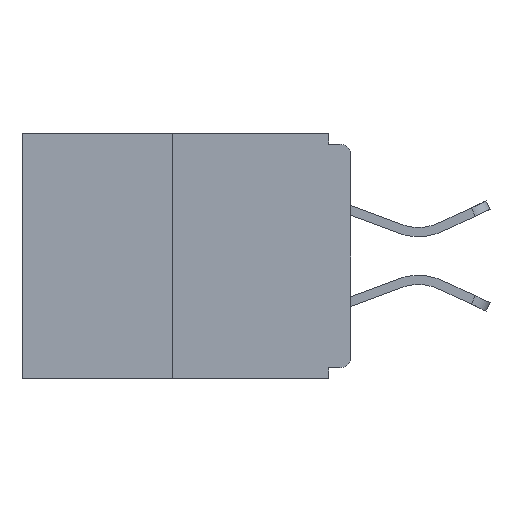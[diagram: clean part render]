
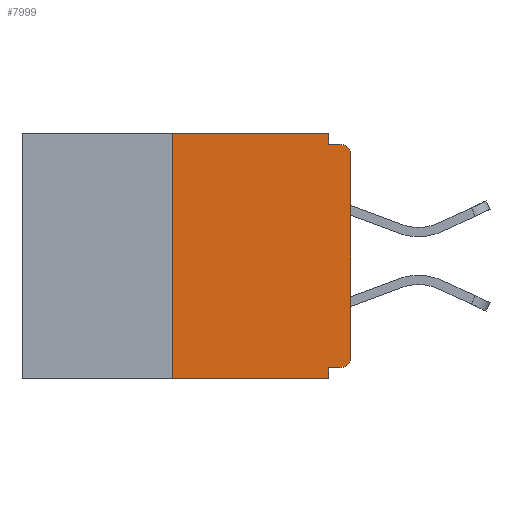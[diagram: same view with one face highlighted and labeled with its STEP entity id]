
A CAD part, left-side view. The second image highlights one B-rep face of the part: STEP entity #7999.
In plain terms, the highlighted planar face has unit normal (-1, 0, 0).
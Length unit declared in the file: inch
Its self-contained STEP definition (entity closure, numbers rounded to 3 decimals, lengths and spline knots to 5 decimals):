
#381 = CARTESIAN_POINT ( 'NONE',  ( 0., 0., 0. ) ) ;
#483 = EDGE_CURVE ( 'NONE', #3316, #15948, #10202, .T. ) ;
#600 = DIRECTION ( 'NONE',  ( -1., 0., 0. ) ) ;
#692 = LINE ( 'NONE', #10729, #14677 ) ;
#743 = CARTESIAN_POINT ( 'NONE',  ( 0., 0., -0.03 ) ) ;
#961 = ORIENTED_EDGE ( 'NONE', *, *, #10037, .F. ) ;
#969 = AXIS2_PLACEMENT_3D ( 'NONE', #8004, #9187, #3056 ) ;
#1356 = CIRCLE ( 'NONE', #11951, 0.015 ) ;
#1617 = VECTOR ( 'NONE', #6879, 39.37008 ) ;
#1692 = CARTESIAN_POINT ( 'NONE',  ( 0., 0.25, 0. ) ) ;
#2631 = DIRECTION ( 'NONE',  ( 0., -1., 0. ) ) ;
#2662 = ORIENTED_EDGE ( 'NONE', *, *, #15430, .T. ) ;
#3056 = DIRECTION ( 'NONE',  ( 0., 0., -1. ) ) ;
#3062 = EDGE_CURVE ( 'NONE', #14717, #14843, #15489, .T. ) ;
#3171 = LINE ( 'NONE', #15654, #1617 ) ;
#3316 = VERTEX_POINT ( 'NONE', #9797 ) ;
#3442 = EDGE_CURVE ( 'NONE', #5687, #5184, #4719, .T. ) ;
#4093 = VERTEX_POINT ( 'NONE', #1692 ) ;
#4639 = DIRECTION ( 'NONE',  ( 0., 0., -1. ) ) ;
#4719 = LINE ( 'NONE', #381, #10356 ) ;
#4804 = ORIENTED_EDGE ( 'NONE', *, *, #483, .T. ) ;
#5184 = VERTEX_POINT ( 'NONE', #743 ) ;
#5310 = CARTESIAN_POINT ( 'NONE',  ( 0., 0.031, -0.015 ) ) ;
#5315 = DIRECTION ( 'NONE',  ( 0., -1., 0. ) ) ;
#5323 = ORIENTED_EDGE ( 'NONE', *, *, #12602, .F. ) ;
#5418 = CARTESIAN_POINT ( 'NONE',  ( 0., 0.46, -0.343 ) ) ;
#5457 = VECTOR ( 'NONE', #2631, 39.37008 ) ;
#5539 = EDGE_CURVE ( 'NONE', #5184, #14843, #1356, .T. ) ;
#5683 = CIRCLE ( 'NONE', #969, 0.015 ) ;
#5687 = VERTEX_POINT ( 'NONE', #11135 ) ;
#6477 = CARTESIAN_POINT ( 'NONE',  ( 0., 0.031, -0.343 ) ) ;
#6554 = CARTESIAN_POINT ( 'NONE',  ( 0., 0., -0.328 ) ) ;
#6836 = ORIENTED_EDGE ( 'NONE', *, *, #5539, .T. ) ;
#6879 = DIRECTION ( 'NONE',  ( 0., 0., -1. ) ) ;
#7181 = CARTESIAN_POINT ( 'NONE',  ( 0., 0.015, -0.328 ) ) ;
#7655 = VECTOR ( 'NONE', #10045, 39.37008 ) ;
#7786 = CARTESIAN_POINT ( 'NONE',  ( 0., 0.46, 0. ) ) ;
#7956 = DIRECTION ( 'NONE',  ( 0., 0., -1. ) ) ;
#7999 = ADVANCED_FACE ( 'NONE', ( #14694 ), #13036, .F. ) ;
#8004 = CARTESIAN_POINT ( 'NONE',  ( 0., 0.015, -0.313 ) ) ;
#8194 = VECTOR ( 'NONE', #14007, 39.37008 ) ;
#8277 = CARTESIAN_POINT ( 'NONE',  ( 0., 0.031, 0. ) ) ;
#9087 = CARTESIAN_POINT ( 'NONE',  ( 0., 0., -0.015 ) ) ;
#9134 = EDGE_LOOP ( 'NONE', ( #5323, #9740, #4804, #13266, #10507, #2662, #14422, #6836, #13509, #961 ) ) ;
#9187 = DIRECTION ( 'NONE',  ( -1., 0., 0. ) ) ;
#9358 = VERTEX_POINT ( 'NONE', #13633 ) ;
#9740 = ORIENTED_EDGE ( 'NONE', *, *, #10738, .F. ) ;
#9797 = CARTESIAN_POINT ( 'NONE',  ( 0., 0.25, -0.343 ) ) ;
#10026 = DIRECTION ( 'NONE',  ( 0., 0., 1. ) ) ;
#10037 = EDGE_CURVE ( 'NONE', #13967, #14717, #692, .T. ) ;
#10045 = DIRECTION ( 'NONE',  ( 0., -1., 0. ) ) ;
#10202 = LINE ( 'NONE', #5418, #13933 ) ;
#10356 = VECTOR ( 'NONE', #12655, 39.37008 ) ;
#10507 = ORIENTED_EDGE ( 'NONE', *, *, #14682, .F. ) ;
#10713 = LINE ( 'NONE', #6554, #8194 ) ;
#10729 = CARTESIAN_POINT ( 'NONE',  ( 0., 0.031, 0. ) ) ;
#10738 = EDGE_CURVE ( 'NONE', #3316, #4093, #11344, .T. ) ;
#11135 = CARTESIAN_POINT ( 'NONE',  ( 0., 0., -0.313 ) ) ;
#11216 = CARTESIAN_POINT ( 'NONE',  ( 0., 0.25, 0. ) ) ;
#11344 = LINE ( 'NONE', #11216, #15078 ) ;
#11631 = DIRECTION ( 'NONE',  ( 1., 0., 0. ) ) ;
#11951 = AXIS2_PLACEMENT_3D ( 'NONE', #13206, #600, #14296 ) ;
#12235 = CARTESIAN_POINT ( 'NONE',  ( 0., 0.015, -0.015 ) ) ;
#12602 = EDGE_CURVE ( 'NONE', #4093, #13967, #13630, .T. ) ;
#12655 = DIRECTION ( 'NONE',  ( 0., 0., 1. ) ) ;
#13036 = PLANE ( 'NONE',  #15024 ) ;
#13073 = VERTEX_POINT ( 'NONE', #7181 ) ;
#13206 = CARTESIAN_POINT ( 'NONE',  ( 0., 0.015, -0.03 ) ) ;
#13266 = ORIENTED_EDGE ( 'NONE', *, *, #15551, .F. ) ;
#13509 = ORIENTED_EDGE ( 'NONE', *, *, #3062, .F. ) ;
#13630 = LINE ( 'NONE', #15101, #5457 ) ;
#13633 = CARTESIAN_POINT ( 'NONE',  ( 0., 0.031, -0.328 ) ) ;
#13933 = VECTOR ( 'NONE', #5315, 39.37008 ) ;
#13967 = VERTEX_POINT ( 'NONE', #8277 ) ;
#14007 = DIRECTION ( 'NONE',  ( 0., 1., 0. ) ) ;
#14296 = DIRECTION ( 'NONE',  ( 0., 0., -1. ) ) ;
#14422 = ORIENTED_EDGE ( 'NONE', *, *, #3442, .T. ) ;
#14677 = VECTOR ( 'NONE', #4639, 39.37008 ) ;
#14682 = EDGE_CURVE ( 'NONE', #13073, #9358, #10713, .T. ) ;
#14694 = FACE_OUTER_BOUND ( 'NONE', #9134, .T. ) ;
#14717 = VERTEX_POINT ( 'NONE', #5310 ) ;
#14843 = VERTEX_POINT ( 'NONE', #12235 ) ;
#15024 = AXIS2_PLACEMENT_3D ( 'NONE', #7786, #11631, #7956 ) ;
#15078 = VECTOR ( 'NONE', #10026, 39.37008 ) ;
#15101 = CARTESIAN_POINT ( 'NONE',  ( 0., 0.46, 0. ) ) ;
#15430 = EDGE_CURVE ( 'NONE', #13073, #5687, #5683, .T. ) ;
#15489 = LINE ( 'NONE', #9087, #7655 ) ;
#15551 = EDGE_CURVE ( 'NONE', #9358, #15948, #3171, .T. ) ;
#15654 = CARTESIAN_POINT ( 'NONE',  ( 0., 0.031, -0.343 ) ) ;
#15948 = VERTEX_POINT ( 'NONE', #6477 ) ;
